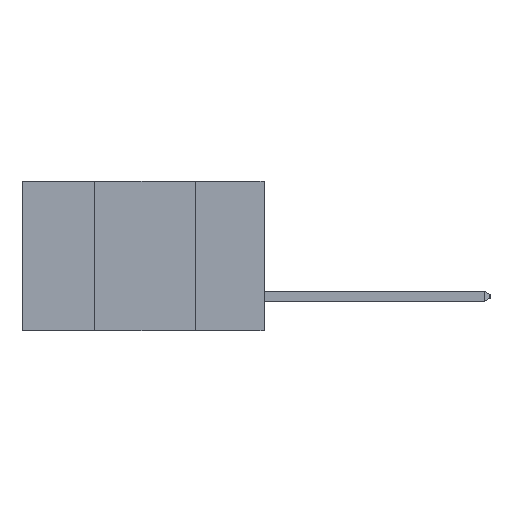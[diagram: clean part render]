
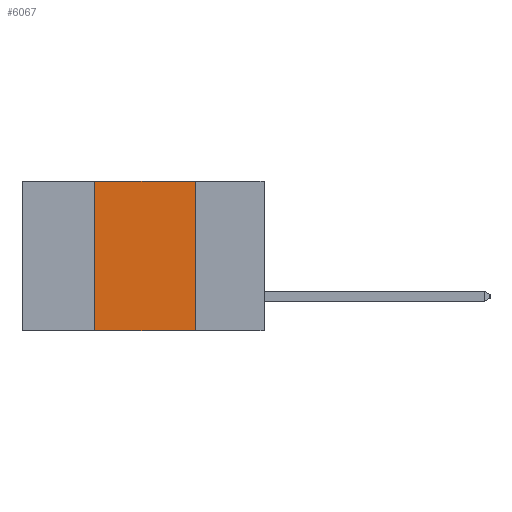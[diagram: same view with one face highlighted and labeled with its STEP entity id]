
A CAD part, left-side view. The second image highlights one B-rep face of the part: STEP entity #6067.
In plain terms, the highlighted planar face has unit normal (-1, 0, 0).
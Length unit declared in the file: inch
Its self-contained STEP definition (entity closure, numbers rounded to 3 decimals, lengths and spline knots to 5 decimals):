
#428 = VECTOR ( 'NONE', #10151, 39.37008 ) ;
#2410 = EDGE_CURVE ( 'NONE', #8337, #7150, #19482, .T. ) ;
#3257 = CARTESIAN_POINT ( 'NONE',  ( 0., 0.17, 0. ) ) ;
#3611 = ORIENTED_EDGE ( 'NONE', *, *, #2410, .T. ) ;
#3894 = EDGE_CURVE ( 'NONE', #8337, #8293, #6012, .T. ) ;
#6012 = LINE ( 'NONE', #14732, #17509 ) ;
#6067 = ADVANCED_FACE ( 'NONE', ( #14041 ), #12361, .F. ) ;
#7150 = VERTEX_POINT ( 'NONE', #11977 ) ;
#8293 = VERTEX_POINT ( 'NONE', #14794 ) ;
#8337 = VERTEX_POINT ( 'NONE', #13421 ) ;
#8628 = CARTESIAN_POINT ( 'NONE',  ( 0., 0.17, -0.37 ) ) ;
#9338 = VECTOR ( 'NONE', #18770, 39.37008 ) ;
#10151 = DIRECTION ( 'NONE',  ( 0., 0., -1. ) ) ;
#10399 = EDGE_LOOP ( 'NONE', ( #10436, #10902, #18669, #3611 ) ) ;
#10436 = ORIENTED_EDGE ( 'NONE', *, *, #17413, .F. ) ;
#10902 = ORIENTED_EDGE ( 'NONE', *, *, #16229, .F. ) ;
#11472 = CARTESIAN_POINT ( 'NONE',  ( 0., 0.6, 0. ) ) ;
#11977 = CARTESIAN_POINT ( 'NONE',  ( 0., 0.17, -0.37 ) ) ;
#12147 = DIRECTION ( 'NONE',  ( 0., 0., -1. ) ) ;
#12174 = DIRECTION ( 'NONE',  ( 1., 0., 0. ) ) ;
#12255 = CARTESIAN_POINT ( 'NONE',  ( 0., 0.6, 0. ) ) ;
#12361 = PLANE ( 'NONE',  #17250 ) ;
#12837 = LINE ( 'NONE', #8628, #428 ) ;
#13421 = CARTESIAN_POINT ( 'NONE',  ( 0., 0.42, -0.37 ) ) ;
#14041 = FACE_OUTER_BOUND ( 'NONE', #10399, .T. ) ;
#14522 = DIRECTION ( 'NONE',  ( 0., 0., 1. ) ) ;
#14732 = CARTESIAN_POINT ( 'NONE',  ( 0., 0.42, -0.37 ) ) ;
#14794 = CARTESIAN_POINT ( 'NONE',  ( 0., 0.42, 0. ) ) ;
#15288 = DIRECTION ( 'NONE',  ( 0., -1., 0. ) ) ;
#15720 = CARTESIAN_POINT ( 'NONE',  ( 0., 0.6, -0.37 ) ) ;
#15754 = VECTOR ( 'NONE', #15288, 39.37008 ) ;
#16229 = EDGE_CURVE ( 'NONE', #8293, #17260, #17217, .T. ) ;
#17217 = LINE ( 'NONE', #11472, #9338 ) ;
#17250 = AXIS2_PLACEMENT_3D ( 'NONE', #12255, #12174, #12147 ) ;
#17260 = VERTEX_POINT ( 'NONE', #3257 ) ;
#17413 = EDGE_CURVE ( 'NONE', #17260, #7150, #12837, .T. ) ;
#17509 = VECTOR ( 'NONE', #14522, 39.37008 ) ;
#18669 = ORIENTED_EDGE ( 'NONE', *, *, #3894, .F. ) ;
#18770 = DIRECTION ( 'NONE',  ( 0., -1., 0. ) ) ;
#19482 = LINE ( 'NONE', #15720, #15754 ) ;
